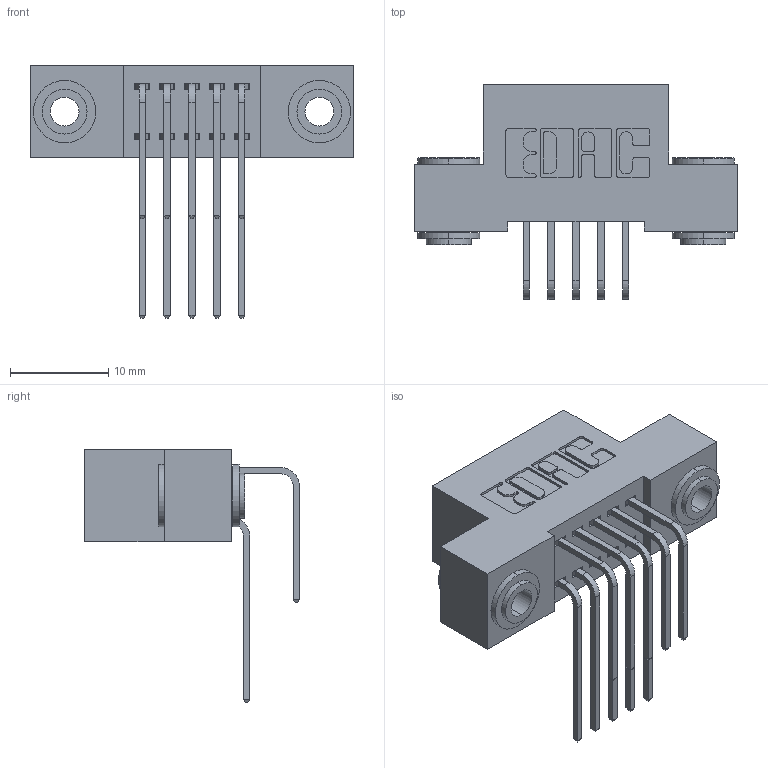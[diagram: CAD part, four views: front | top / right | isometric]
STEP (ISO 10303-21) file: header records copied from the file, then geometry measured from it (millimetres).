
FILE_DESCRIPTION (( 'STEP AP203' ), '1' );
FILE_NAME ('342-010-558-203.STEP', '2019-10-01T14:48:15', ( '' ), ( '' ), 'SwSTEP 2.0', 'SolidWorks 2016', '' );
FILE_SCHEMA (( 'CONFIG_CONTROL_DESIGN' ));
Length unit declared in the file: inch
Products named in the file (5): 342 Part_.156 TH; 345-292-001_558 559 Tail - 1; 345-292-001_558 Tail - 2; 342-250-002_345-250-002-102; 342-010-558-203
Assembly tree (13 placements, depth 2):
  342-010-558-203
    342 Part_.156 TH
    345-292-001_558 559 Tail - 1  x5
    345-292-001_558 Tail - 2  x5
    342-250-002_345-250-002-102  x2
Bounding box: 33.02 x 21.91 x 25.78 mm (x, y, z)
Volume: 2872.2 mm3; surface area: 4238.6 mm2
Topology: 13 solids, 13 shells, 688 faces, 1985 edges, 1306 vertices
Faces by surface type: plane 456, cylinder 224, cone 8
Entity records: 10304 total; most frequent: CARTESIAN_POINT 1776, ORIENTED_EDGE 1654, DIRECTION 1597, EDGE_CURVE 827, LINE 635, VECTOR 635, VERTEX_POINT 546, AXIS2_PLACEMENT_3D 481
